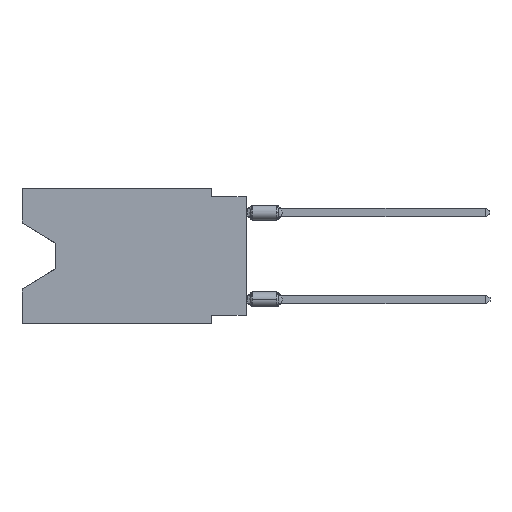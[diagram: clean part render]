
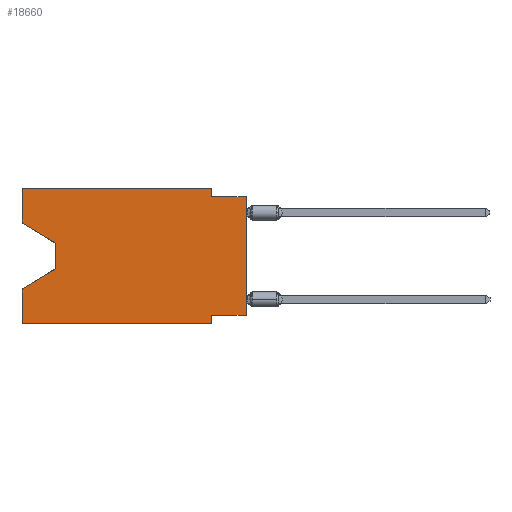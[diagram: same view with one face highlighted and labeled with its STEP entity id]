
A CAD part, left-side view. The second image highlights one B-rep face of the part: STEP entity #18660.
In plain terms, the highlighted planar face has unit normal (-1, 0, 0).
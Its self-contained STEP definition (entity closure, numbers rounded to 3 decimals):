
#33 = ORIENTED_EDGE ( 'NONE', *, *, #7969, .F. ) ;
#291 = VECTOR ( 'NONE', #9186, 1000. ) ;
#302 = CARTESIAN_POINT ( 'NONE',  ( 0., 0., -0.635 ) ) ;
#343 = LINE ( 'NONE', #24035, #9221 ) ;
#391 = LINE ( 'NONE', #4395, #3610 ) ;
#1066 = CARTESIAN_POINT ( 'NONE',  ( 0., 16.383, 0. ) ) ;
#1091 = EDGE_LOOP ( 'NONE', ( #4441, #18240, #8423, #23051, #24715, #14600, #18713, #1644, #16660, #33, #11216, #22877 ) ) ;
#1457 = LINE ( 'NONE', #1066, #20226 ) ;
#1644 = ORIENTED_EDGE ( 'NONE', *, *, #20801, .T. ) ;
#2779 = EDGE_CURVE ( 'NONE', #22387, #9877, #3540, .T. ) ;
#3141 = CARTESIAN_POINT ( 'NONE',  ( 0., 13.97, -4.013 ) ) ;
#3189 = VERTEX_POINT ( 'NONE', #11277 ) ;
#3540 = LINE ( 'NONE', #17019, #4796 ) ;
#3610 = VECTOR ( 'NONE', #8268, 1000. ) ;
#3892 = CARTESIAN_POINT ( 'NONE',  ( 0., 16.383, 0. ) ) ;
#3980 = EDGE_CURVE ( 'NONE', #25234, #16618, #391, .T. ) ;
#4340 = DIRECTION ( 'NONE',  ( 0., 1., 0. ) ) ;
#4395 = CARTESIAN_POINT ( 'NONE',  ( 0., 13.97, -4.013 ) ) ;
#4441 = ORIENTED_EDGE ( 'NONE', *, *, #13914, .T. ) ;
#4456 = DIRECTION ( 'NONE',  ( 0., 0., 1. ) ) ;
#4759 = EDGE_CURVE ( 'NONE', #9567, #10978, #22557, .T. ) ;
#4796 = VECTOR ( 'NONE', #17156, 1000. ) ;
#5364 = CARTESIAN_POINT ( 'NONE',  ( 0., 16.383, 0. ) ) ;
#5881 = LINE ( 'NONE', #5364, #12151 ) ;
#5943 = VERTEX_POINT ( 'NONE', #16260 ) ;
#6175 = DIRECTION ( 'NONE',  ( 0., 0.855, -0.519 ) ) ;
#6658 = LINE ( 'NONE', #16647, #23681 ) ;
#6841 = LINE ( 'NONE', #16215, #12651 ) ;
#7969 = EDGE_CURVE ( 'NONE', #22147, #9567, #6841, .T. ) ;
#8163 = EDGE_CURVE ( 'NONE', #20161, #9877, #11122, .T. ) ;
#8268 = DIRECTION ( 'NONE',  ( 0., 0., -1. ) ) ;
#8270 = CARTESIAN_POINT ( 'NONE',  ( 0., 2.54, -0.635 ) ) ;
#8423 = ORIENTED_EDGE ( 'NONE', *, *, #12190, .T. ) ;
#8774 = LINE ( 'NONE', #18392, #17690 ) ;
#8849 = CARTESIAN_POINT ( 'NONE',  ( 0., 2.54, -9.271 ) ) ;
#9186 = DIRECTION ( 'NONE',  ( 0., -1., 0. ) ) ;
#9221 = VECTOR ( 'NONE', #4340, 1000. ) ;
#9355 = DIRECTION ( 'NONE',  ( 0., -0.855, -0.519 ) ) ;
#9359 = DIRECTION ( 'NONE',  ( 0., 0., 1. ) ) ;
#9504 = EDGE_CURVE ( 'NONE', #5943, #22147, #8774, .T. ) ;
#9567 = VERTEX_POINT ( 'NONE', #8270 ) ;
#9590 = DIRECTION ( 'NONE',  ( 1., 0., 0. ) ) ;
#9877 = VERTEX_POINT ( 'NONE', #19671 ) ;
#10978 = VERTEX_POINT ( 'NONE', #19160 ) ;
#11122 = LINE ( 'NONE', #17236, #291 ) ;
#11216 = ORIENTED_EDGE ( 'NONE', *, *, #9504, .F. ) ;
#11277 = CARTESIAN_POINT ( 'NONE',  ( 0., 0., -9.271 ) ) ;
#11312 = VERTEX_POINT ( 'NONE', #20929 ) ;
#12151 = VECTOR ( 'NONE', #21711, 1000. ) ;
#12190 = EDGE_CURVE ( 'NONE', #16618, #21244, #6658, .T. ) ;
#12651 = VECTOR ( 'NONE', #22429, 1000. ) ;
#12661 = DIRECTION ( 'NONE',  ( 0., -1., 0. ) ) ;
#13047 = CARTESIAN_POINT ( 'NONE',  ( 0., 16.383, -9.906 ) ) ;
#13423 = CARTESIAN_POINT ( 'NONE',  ( 0., 2.54, 0. ) ) ;
#13914 = EDGE_CURVE ( 'NONE', #11312, #25234, #19220, .T. ) ;
#14148 = DIRECTION ( 'NONE',  ( 0., -1., 0. ) ) ;
#14600 = ORIENTED_EDGE ( 'NONE', *, *, #2779, .F. ) ;
#15552 = FACE_OUTER_BOUND ( 'NONE', #1091, .T. ) ;
#16215 = CARTESIAN_POINT ( 'NONE',  ( 0., 2.54, 0. ) ) ;
#16260 = CARTESIAN_POINT ( 'NONE',  ( 0., 16.383, 0. ) ) ;
#16618 = VERTEX_POINT ( 'NONE', #17564 ) ;
#16647 = CARTESIAN_POINT ( 'NONE',  ( 0., 13.97, -5.893 ) ) ;
#16660 = ORIENTED_EDGE ( 'NONE', *, *, #4759, .F. ) ;
#17019 = CARTESIAN_POINT ( 'NONE',  ( 0., 2.54, -9.906 ) ) ;
#17156 = DIRECTION ( 'NONE',  ( 0., 0., -1. ) ) ;
#17236 = CARTESIAN_POINT ( 'NONE',  ( 0., 16.383, -9.906 ) ) ;
#17564 = CARTESIAN_POINT ( 'NONE',  ( 0., 13.97, -5.893 ) ) ;
#17690 = VECTOR ( 'NONE', #12661, 1000. ) ;
#17834 = VECTOR ( 'NONE', #4456, 1000. ) ;
#18161 = EDGE_CURVE ( 'NONE', #20161, #21244, #1457, .T. ) ;
#18240 = ORIENTED_EDGE ( 'NONE', *, *, #3980, .T. ) ;
#18392 = CARTESIAN_POINT ( 'NONE',  ( 0., 16.383, 0. ) ) ;
#18660 = ADVANCED_FACE ( 'NONE', ( #15552 ), #19962, .F. ) ;
#18713 = ORIENTED_EDGE ( 'NONE', *, *, #22276, .F. ) ;
#19160 = CARTESIAN_POINT ( 'NONE',  ( 0., 0., -0.635 ) ) ;
#19220 = LINE ( 'NONE', #24628, #25192 ) ;
#19671 = CARTESIAN_POINT ( 'NONE',  ( 0., 2.54, -9.906 ) ) ;
#19962 = PLANE ( 'NONE',  #25176 ) ;
#20161 = VERTEX_POINT ( 'NONE', #13047 ) ;
#20226 = VECTOR ( 'NONE', #9359, 1000. ) ;
#20273 = CARTESIAN_POINT ( 'NONE',  ( 0., 0., 0. ) ) ;
#20801 = EDGE_CURVE ( 'NONE', #3189, #10978, #21977, .T. ) ;
#20929 = CARTESIAN_POINT ( 'NONE',  ( 0., 16.383, -2.546 ) ) ;
#21244 = VERTEX_POINT ( 'NONE', #22801 ) ;
#21711 = DIRECTION ( 'NONE',  ( 0., 0., 1. ) ) ;
#21786 = DIRECTION ( 'NONE',  ( 0., 0., -1. ) ) ;
#21977 = LINE ( 'NONE', #20273, #17834 ) ;
#22147 = VERTEX_POINT ( 'NONE', #13423 ) ;
#22276 = EDGE_CURVE ( 'NONE', #3189, #22387, #343, .T. ) ;
#22387 = VERTEX_POINT ( 'NONE', #8849 ) ;
#22429 = DIRECTION ( 'NONE',  ( 0., 0., -1. ) ) ;
#22557 = LINE ( 'NONE', #302, #23743 ) ;
#22801 = CARTESIAN_POINT ( 'NONE',  ( 0., 16.383, -7.36 ) ) ;
#22877 = ORIENTED_EDGE ( 'NONE', *, *, #23876, .F. ) ;
#23051 = ORIENTED_EDGE ( 'NONE', *, *, #18161, .F. ) ;
#23681 = VECTOR ( 'NONE', #6175, 1000. ) ;
#23743 = VECTOR ( 'NONE', #14148, 1000. ) ;
#23876 = EDGE_CURVE ( 'NONE', #11312, #5943, #5881, .T. ) ;
#24035 = CARTESIAN_POINT ( 'NONE',  ( 0., 0., -9.271 ) ) ;
#24628 = CARTESIAN_POINT ( 'NONE',  ( 0., 16.383, -2.546 ) ) ;
#24715 = ORIENTED_EDGE ( 'NONE', *, *, #8163, .T. ) ;
#25176 = AXIS2_PLACEMENT_3D ( 'NONE', #3892, #9590, #21786 ) ;
#25192 = VECTOR ( 'NONE', #9355, 1000. ) ;
#25234 = VERTEX_POINT ( 'NONE', #3141 ) ;
